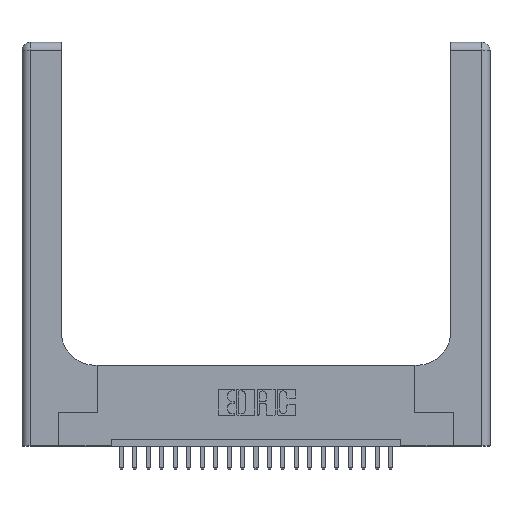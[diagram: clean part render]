
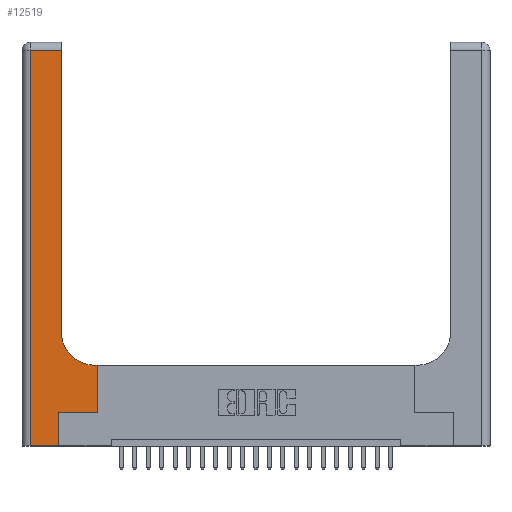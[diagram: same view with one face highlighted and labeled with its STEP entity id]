
A CAD part, top view. The second image highlights one B-rep face of the part: STEP entity #12519.
In plain terms, the highlighted planar face has unit normal (0, 0, 1).
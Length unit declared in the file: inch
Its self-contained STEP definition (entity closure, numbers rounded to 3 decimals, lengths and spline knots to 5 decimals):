
#575 = ORIENTED_EDGE ( 'NONE', *, *, #5651, .T. ) ;
#625 = LINE ( 'NONE', #21071, #23772 ) ;
#1017 = LINE ( 'NONE', #7937, #20113 ) ;
#1337 = LINE ( 'NONE', #23271, #16103 ) ;
#2807 = CARTESIAN_POINT ( 'NONE',  ( 0.06, 0., 0.37 ) ) ;
#2813 = EDGE_CURVE ( 'NONE', #9490, #11291, #19915, .T. ) ;
#2907 = DIRECTION ( 'NONE',  ( -1., 0., 0. ) ) ;
#3078 = ORIENTED_EDGE ( 'NONE', *, *, #2813, .T. ) ;
#4027 = ORIENTED_EDGE ( 'NONE', *, *, #19136, .T. ) ;
#4786 = DIRECTION ( 'NONE',  ( 0., -1., 0. ) ) ;
#4862 = CARTESIAN_POINT ( 'NONE',  ( 0.2915, 2.94, 0.37 ) ) ;
#5651 = EDGE_CURVE ( 'NONE', #15959, #9128, #625, .T. ) ;
#5860 = ORIENTED_EDGE ( 'NONE', *, *, #13064, .T. ) ;
#6147 = PLANE ( 'NONE',  #9144 ) ;
#6289 = VERTEX_POINT ( 'NONE', #17990 ) ;
#6557 = CARTESIAN_POINT ( 'NONE',  ( 0.5585, 0.25, 0.37 ) ) ;
#6626 = EDGE_CURVE ( 'NONE', #16330, #15959, #8367, .T. ) ;
#7333 = CIRCLE ( 'NONE', #10797, 0.25 ) ;
#7387 = VERTEX_POINT ( 'NONE', #4862 ) ;
#7730 = CARTESIAN_POINT ( 'NONE',  ( 0.269, 0.25, 0.37 ) ) ;
#7863 = DIRECTION ( 'NONE',  ( 1., 0., 0. ) ) ;
#7937 = CARTESIAN_POINT ( 'NONE',  ( 0.269, 0.25, 0.37 ) ) ;
#8208 = EDGE_CURVE ( 'NONE', #11291, #20162, #18774, .T. ) ;
#8210 = FACE_OUTER_BOUND ( 'NONE', #14553, .T. ) ;
#8365 = DIRECTION ( 'NONE',  ( 0., 1., 0. ) ) ;
#8367 = LINE ( 'NONE', #8593, #17098 ) ;
#8593 = CARTESIAN_POINT ( 'NONE',  ( 0., 0., 0.37 ) ) ;
#9128 = VERTEX_POINT ( 'NONE', #7730 ) ;
#9144 = AXIS2_PLACEMENT_3D ( 'NONE', #22696, #19010, #15284 ) ;
#9490 = VERTEX_POINT ( 'NONE', #10591 ) ;
#9629 = ORIENTED_EDGE ( 'NONE', *, *, #19351, .T. ) ;
#10432 = CARTESIAN_POINT ( 'NONE',  ( 0.269, 0., 0.37 ) ) ;
#10591 = CARTESIAN_POINT ( 'NONE',  ( 0.5585, 0.25, 0.37 ) ) ;
#10797 = AXIS2_PLACEMENT_3D ( 'NONE', #16503, #10805, #14397 ) ;
#10805 = DIRECTION ( 'NONE',  ( 0., 0., -1. ) ) ;
#11128 = VECTOR ( 'NONE', #16882, 39.37008 ) ;
#11291 = VERTEX_POINT ( 'NONE', #20167 ) ;
#12264 = EDGE_CURVE ( 'NONE', #22785, #16330, #1337, .T. ) ;
#12325 = DIRECTION ( 'NONE',  ( 1., 0., 0. ) ) ;
#12519 = ADVANCED_FACE ( 'NONE', ( #8210 ), #6147, .F. ) ;
#13064 = EDGE_CURVE ( 'NONE', #6289, #7387, #22157, .T. ) ;
#14086 = CARTESIAN_POINT ( 'NONE',  ( 0.2915, 0.6, 0.37 ) ) ;
#14397 = DIRECTION ( 'NONE',  ( 1., 0., 0. ) ) ;
#14553 = EDGE_LOOP ( 'NONE', ( #5860, #18416, #22045, #18278, #575, #9629, #3078, #20611, #4027 ) ) ;
#14560 = CARTESIAN_POINT ( 'NONE',  ( 0., 2.94, 0.37 ) ) ;
#14934 = CARTESIAN_POINT ( 'NONE',  ( 0.2915, 3., 0.37 ) ) ;
#15284 = DIRECTION ( 'NONE',  ( -1., 0., 0. ) ) ;
#15346 = LINE ( 'NONE', #14560, #17672 ) ;
#15959 = VERTEX_POINT ( 'NONE', #10432 ) ;
#16103 = VECTOR ( 'NONE', #4786, 39.37008 ) ;
#16330 = VERTEX_POINT ( 'NONE', #2807 ) ;
#16361 = EDGE_CURVE ( 'NONE', #7387, #22785, #15346, .T. ) ;
#16503 = CARTESIAN_POINT ( 'NONE',  ( 0.5415, 0.85, 0.37 ) ) ;
#16549 = CARTESIAN_POINT ( 'NONE',  ( 0.06, 2.94, 0.37 ) ) ;
#16882 = DIRECTION ( 'NONE',  ( 0., 1., 0. ) ) ;
#17051 = DIRECTION ( 'NONE',  ( 0., 1., 0. ) ) ;
#17098 = VECTOR ( 'NONE', #12325, 39.37008 ) ;
#17491 = CARTESIAN_POINT ( 'NONE',  ( 0.5415, 0.6, 0.37 ) ) ;
#17672 = VECTOR ( 'NONE', #23597, 39.37008 ) ;
#17990 = CARTESIAN_POINT ( 'NONE',  ( 0.2915, 0.85, 0.37 ) ) ;
#18278 = ORIENTED_EDGE ( 'NONE', *, *, #6626, .T. ) ;
#18416 = ORIENTED_EDGE ( 'NONE', *, *, #16361, .T. ) ;
#18774 = LINE ( 'NONE', #14086, #20214 ) ;
#19010 = DIRECTION ( 'NONE',  ( 0., 0., -1. ) ) ;
#19136 = EDGE_CURVE ( 'NONE', #20162, #6289, #7333, .T. ) ;
#19337 = VECTOR ( 'NONE', #8365, 39.37008 ) ;
#19351 = EDGE_CURVE ( 'NONE', #9128, #9490, #1017, .T. ) ;
#19915 = LINE ( 'NONE', #6557, #19337 ) ;
#20113 = VECTOR ( 'NONE', #7863, 39.37008 ) ;
#20162 = VERTEX_POINT ( 'NONE', #17491 ) ;
#20167 = CARTESIAN_POINT ( 'NONE',  ( 0.5585, 0.6, 0.37 ) ) ;
#20214 = VECTOR ( 'NONE', #2907, 39.37008 ) ;
#20611 = ORIENTED_EDGE ( 'NONE', *, *, #8208, .T. ) ;
#21071 = CARTESIAN_POINT ( 'NONE',  ( 0.269, 0., 0.37 ) ) ;
#22045 = ORIENTED_EDGE ( 'NONE', *, *, #12264, .T. ) ;
#22157 = LINE ( 'NONE', #14934, #11128 ) ;
#22696 = CARTESIAN_POINT ( 'NONE',  ( 0., 3., 0.37 ) ) ;
#22785 = VERTEX_POINT ( 'NONE', #16549 ) ;
#23271 = CARTESIAN_POINT ( 'NONE',  ( 0.06, 3., 0.37 ) ) ;
#23597 = DIRECTION ( 'NONE',  ( -1., 0., 0. ) ) ;
#23772 = VECTOR ( 'NONE', #17051, 39.37008 ) ;
